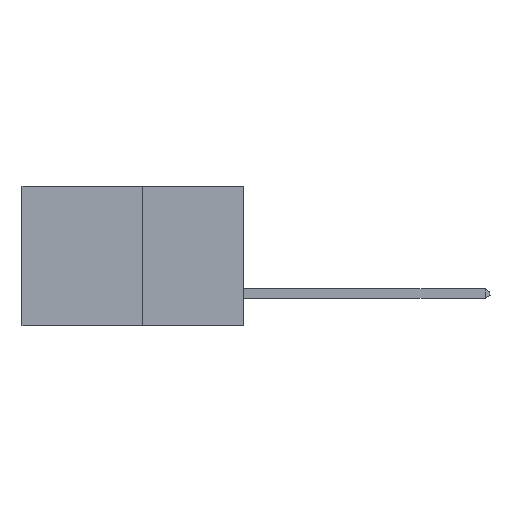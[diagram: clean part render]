
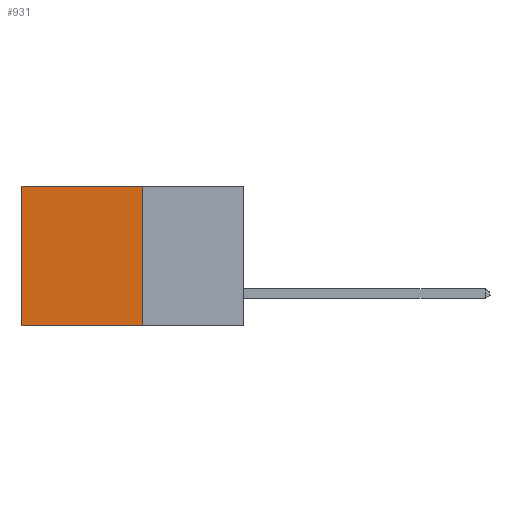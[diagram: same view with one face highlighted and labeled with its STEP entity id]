
A CAD part, left-side view. The second image highlights one B-rep face of the part: STEP entity #931.
In plain terms, the highlighted planar face has unit normal (-1, 0, 0).
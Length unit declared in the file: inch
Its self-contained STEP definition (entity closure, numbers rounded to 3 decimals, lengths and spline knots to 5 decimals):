
#931 = ADVANCED_FACE ( 'NONE', ( #11004 ), #15954, .F. ) ;
#1257 = VECTOR ( 'NONE', #10927, 39.37008 ) ;
#2229 = CARTESIAN_POINT ( 'NONE',  ( 0.277, 0.27, -0.37 ) ) ;
#4310 = VECTOR ( 'NONE', #18931, 39.37008 ) ;
#4709 = VERTEX_POINT ( 'NONE', #10291 ) ;
#5386 = CARTESIAN_POINT ( 'NONE',  ( 0.277, 0.59, 0. ) ) ;
#7741 = ORIENTED_EDGE ( 'NONE', *, *, #20911, .T. ) ;
#8192 = VECTOR ( 'NONE', #10242, 39.37008 ) ;
#8570 = CARTESIAN_POINT ( 'NONE',  ( 0.277, 0.27, 0. ) ) ;
#9524 = VERTEX_POINT ( 'NONE', #16994 ) ;
#9525 = LINE ( 'NONE', #17010, #18246 ) ;
#10033 = VERTEX_POINT ( 'NONE', #11922 ) ;
#10242 = DIRECTION ( 'NONE',  ( 0., 1., 0. ) ) ;
#10291 = CARTESIAN_POINT ( 'NONE',  ( 0.277, 0.27, -0.37 ) ) ;
#10927 = DIRECTION ( 'NONE',  ( 0., 1., 0. ) ) ;
#11004 = FACE_OUTER_BOUND ( 'NONE', #18161, .T. ) ;
#11922 = CARTESIAN_POINT ( 'NONE',  ( 0.277, 0.27, 0. ) ) ;
#14611 = LINE ( 'NONE', #19079, #1257 ) ;
#14898 = EDGE_CURVE ( 'NONE', #10033, #16851, #16438, .T. ) ;
#15154 = CARTESIAN_POINT ( 'NONE',  ( 0.277, 0.27, -0.37 ) ) ;
#15216 = ORIENTED_EDGE ( 'NONE', *, *, #14898, .T. ) ;
#15613 = DIRECTION ( 'NONE',  ( 0., 0., -1. ) ) ;
#15652 = DIRECTION ( 'NONE',  ( 1., 0., 0. ) ) ;
#15954 = PLANE ( 'NONE',  #18587 ) ;
#16438 = LINE ( 'NONE', #8570, #8192 ) ;
#16468 = EDGE_CURVE ( 'NONE', #4709, #9524, #14611, .T. ) ;
#16851 = VERTEX_POINT ( 'NONE', #5386 ) ;
#16994 = CARTESIAN_POINT ( 'NONE',  ( 0.277, 0.59, -0.37 ) ) ;
#17010 = CARTESIAN_POINT ( 'NONE',  ( 0.277, 0.59, -0.37 ) ) ;
#17562 = LINE ( 'NONE', #2229, #4310 ) ;
#18161 = EDGE_LOOP ( 'NONE', ( #7741, #18508, #18723, #15216 ) ) ;
#18246 = VECTOR ( 'NONE', #18652, 39.37008 ) ;
#18508 = ORIENTED_EDGE ( 'NONE', *, *, #16468, .F. ) ;
#18587 = AXIS2_PLACEMENT_3D ( 'NONE', #15154, #15652, #15613 ) ;
#18652 = DIRECTION ( 'NONE',  ( 0., 0., -1. ) ) ;
#18723 = ORIENTED_EDGE ( 'NONE', *, *, #18845, .F. ) ;
#18845 = EDGE_CURVE ( 'NONE', #10033, #4709, #17562, .T. ) ;
#18931 = DIRECTION ( 'NONE',  ( 0., 0., -1. ) ) ;
#19079 = CARTESIAN_POINT ( 'NONE',  ( 0.277, 0.27, -0.37 ) ) ;
#20911 = EDGE_CURVE ( 'NONE', #16851, #9524, #9525, .T. ) ;
